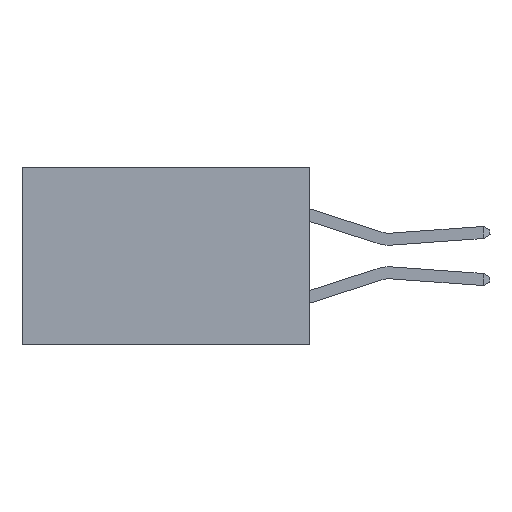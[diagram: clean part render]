
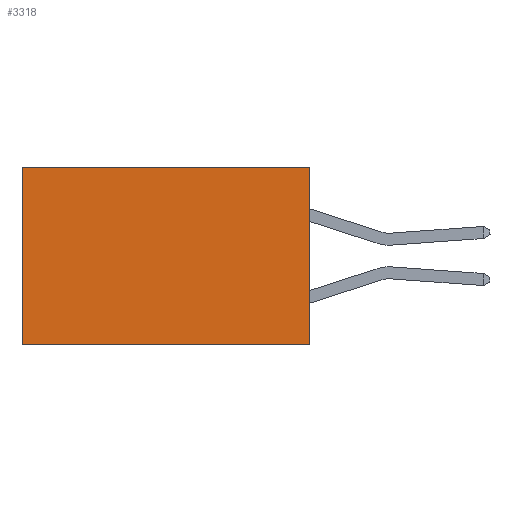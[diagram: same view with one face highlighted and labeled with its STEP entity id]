
A CAD part, left-side view. The second image highlights one B-rep face of the part: STEP entity #3318.
In plain terms, the highlighted planar face has unit normal (-1, 0, 0).
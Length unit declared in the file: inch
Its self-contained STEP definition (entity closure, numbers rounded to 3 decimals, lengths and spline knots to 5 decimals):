
#292 = VECTOR ( 'NONE', #6139, 39.37008 ) ;
#615 = CARTESIAN_POINT ( 'NONE',  ( 0.2615, 0.6, 0. ) ) ;
#830 = EDGE_CURVE ( 'NONE', #1182, #10726, #9928, .T. ) ;
#1182 = VERTEX_POINT ( 'NONE', #5389 ) ;
#1825 = VERTEX_POINT ( 'NONE', #615 ) ;
#1982 = VECTOR ( 'NONE', #7794, 39.37008 ) ;
#2307 = ORIENTED_EDGE ( 'NONE', *, *, #2828, .F. ) ;
#2321 = VERTEX_POINT ( 'NONE', #10659 ) ;
#2828 = EDGE_CURVE ( 'NONE', #2321, #1182, #3838, .T. ) ;
#3318 = ADVANCED_FACE ( 'NONE', ( #6754 ), #8658, .F. ) ;
#3838 = LINE ( 'NONE', #10604, #1982 ) ;
#4779 = CARTESIAN_POINT ( 'NONE',  ( 0.2615, 0., -0.37 ) ) ;
#5389 = CARTESIAN_POINT ( 'NONE',  ( 0.2615, 0., -0.37 ) ) ;
#5492 = CARTESIAN_POINT ( 'NONE',  ( 0.2615, 0.6, -0.37 ) ) ;
#6139 = DIRECTION ( 'NONE',  ( 0., 1., 0. ) ) ;
#6754 = FACE_OUTER_BOUND ( 'NONE', #8083, .T. ) ;
#6870 = AXIS2_PLACEMENT_3D ( 'NONE', #4779, #12944, #9959 ) ;
#7103 = CARTESIAN_POINT ( 'NONE',  ( 0.2615, 0., -0.37 ) ) ;
#7794 = DIRECTION ( 'NONE',  ( 0., 0., -1. ) ) ;
#8083 = EDGE_LOOP ( 'NONE', ( #9995, #12003, #2307, #8305 ) ) ;
#8284 = LINE ( 'NONE', #10487, #11551 ) ;
#8305 = ORIENTED_EDGE ( 'NONE', *, *, #12452, .T. ) ;
#8352 = DIRECTION ( 'NONE',  ( 0., 0., -1. ) ) ;
#8658 = PLANE ( 'NONE',  #6870 ) ;
#9115 = CARTESIAN_POINT ( 'NONE',  ( 0.2615, 0., 0. ) ) ;
#9198 = EDGE_CURVE ( 'NONE', #1825, #10726, #8284, .T. ) ;
#9242 = LINE ( 'NONE', #9115, #292 ) ;
#9928 = LINE ( 'NONE', #7103, #12765 ) ;
#9959 = DIRECTION ( 'NONE',  ( 0., 0., -1. ) ) ;
#9995 = ORIENTED_EDGE ( 'NONE', *, *, #9198, .T. ) ;
#10487 = CARTESIAN_POINT ( 'NONE',  ( 0.2615, 0.6, -0.37 ) ) ;
#10604 = CARTESIAN_POINT ( 'NONE',  ( 0.2615, 0., -0.37 ) ) ;
#10659 = CARTESIAN_POINT ( 'NONE',  ( 0.2615, 0., 0. ) ) ;
#10726 = VERTEX_POINT ( 'NONE', #5492 ) ;
#11103 = DIRECTION ( 'NONE',  ( 0., 1., 0. ) ) ;
#11551 = VECTOR ( 'NONE', #8352, 39.37008 ) ;
#12003 = ORIENTED_EDGE ( 'NONE', *, *, #830, .F. ) ;
#12452 = EDGE_CURVE ( 'NONE', #2321, #1825, #9242, .T. ) ;
#12765 = VECTOR ( 'NONE', #11103, 39.37008 ) ;
#12944 = DIRECTION ( 'NONE',  ( 1., 0., 0. ) ) ;
